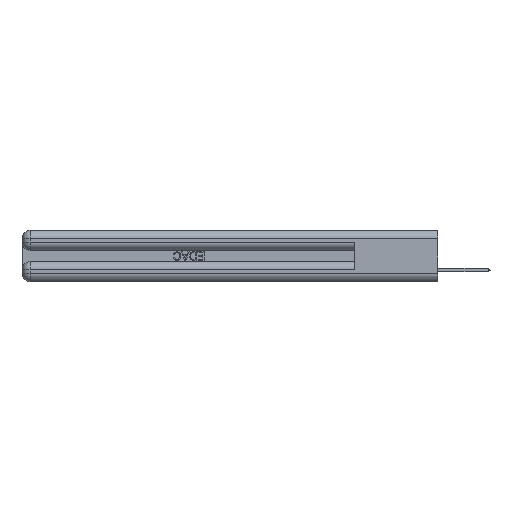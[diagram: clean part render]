
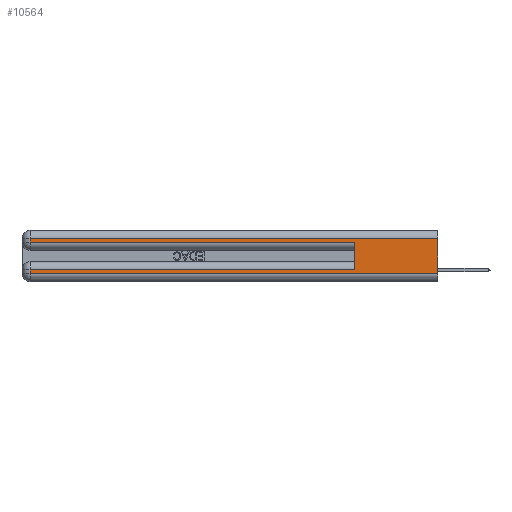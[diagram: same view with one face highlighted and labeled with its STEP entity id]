
A CAD part, left-side view. The second image highlights one B-rep face of the part: STEP entity #10564.
In plain terms, the highlighted planar face has unit normal (-1, 0, 0).
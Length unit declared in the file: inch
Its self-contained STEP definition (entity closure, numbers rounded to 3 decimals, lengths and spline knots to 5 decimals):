
#47 = VERTEX_POINT ( 'NONE', #4497 ) ;
#185 = EDGE_CURVE ( 'NONE', #15919, #32725, #11537, .T. ) ;
#721 = VERTEX_POINT ( 'NONE', #812 ) ;
#812 = CARTESIAN_POINT ( 'NONE',  ( 0., 0., 0.31 ) ) ;
#1434 = CARTESIAN_POINT ( 'NONE',  ( 0., 0., 0.31 ) ) ;
#1485 = VERTEX_POINT ( 'NONE', #38737 ) ;
#2323 = EDGE_CURVE ( 'NONE', #20501, #1485, #36766, .T. ) ;
#4497 = CARTESIAN_POINT ( 'NONE',  ( 0., 0., 0.06 ) ) ;
#5321 = VECTOR ( 'NONE', #28325, 39.37008 ) ;
#5468 = CARTESIAN_POINT ( 'NONE',  ( 0., 0., 0.06 ) ) ;
#7299 = LINE ( 'NONE', #14550, #41602 ) ;
#7753 = ORIENTED_EDGE ( 'NONE', *, *, #2323, .F. ) ;
#8168 = CARTESIAN_POINT ( 'NONE',  ( 0., 2.94, 0.085 ) ) ;
#10564 = ADVANCED_FACE ( 'NONE', ( #11035 ), #19225, .F. ) ;
#11035 = FACE_OUTER_BOUND ( 'NONE', #33458, .T. ) ;
#11233 = VECTOR ( 'NONE', #11423, 39.37008 ) ;
#11423 = DIRECTION ( 'NONE',  ( 0., 1., 0. ) ) ;
#11537 = LINE ( 'NONE', #41353, #5321 ) ;
#11681 = DIRECTION ( 'NONE',  ( 0., -1., 0. ) ) ;
#11895 = VERTEX_POINT ( 'NONE', #8168 ) ;
#13113 = CARTESIAN_POINT ( 'NONE',  ( 0., 2.94, 0.37 ) ) ;
#13334 = CARTESIAN_POINT ( 'NONE',  ( 0., 0., 0.285 ) ) ;
#14045 = LINE ( 'NONE', #33644, #32805 ) ;
#14369 = LINE ( 'NONE', #1434, #11233 ) ;
#14550 = CARTESIAN_POINT ( 'NONE',  ( 0., 0., 0.37 ) ) ;
#15776 = ORIENTED_EDGE ( 'NONE', *, *, #29492, .T. ) ;
#15919 = VERTEX_POINT ( 'NONE', #38553 ) ;
#16603 = CARTESIAN_POINT ( 'NONE',  ( 0., 0.6, 0.145 ) ) ;
#17990 = EDGE_CURVE ( 'NONE', #32725, #1485, #39197, .T. ) ;
#18737 = CARTESIAN_POINT ( 'NONE',  ( 0., 2.94, 0.285 ) ) ;
#19164 = VECTOR ( 'NONE', #11681, 39.37008 ) ;
#19225 = PLANE ( 'NONE',  #32962 ) ;
#19966 = ORIENTED_EDGE ( 'NONE', *, *, #39627, .F. ) ;
#20344 = ORIENTED_EDGE ( 'NONE', *, *, #20624, .T. ) ;
#20501 = VERTEX_POINT ( 'NONE', #36701 ) ;
#20624 = EDGE_CURVE ( 'NONE', #20501, #11895, #14045, .T. ) ;
#22515 = ORIENTED_EDGE ( 'NONE', *, *, #185, .T. ) ;
#24666 = VERTEX_POINT ( 'NONE', #39231 ) ;
#28325 = DIRECTION ( 'NONE',  ( 0., 0., -1. ) ) ;
#28877 = CARTESIAN_POINT ( 'NONE',  ( 0., 0., 0.37 ) ) ;
#29492 = EDGE_CURVE ( 'NONE', #721, #15919, #14369, .T. ) ;
#31294 = DIRECTION ( 'NONE',  ( 0., 0., -1. ) ) ;
#31740 = EDGE_CURVE ( 'NONE', #11895, #24666, #31829, .T. ) ;
#31829 = LINE ( 'NONE', #13113, #38002 ) ;
#32338 = ORIENTED_EDGE ( 'NONE', *, *, #31740, .T. ) ;
#32725 = VERTEX_POINT ( 'NONE', #18737 ) ;
#32805 = VECTOR ( 'NONE', #40495, 39.37008 ) ;
#32962 = AXIS2_PLACEMENT_3D ( 'NONE', #28877, #39152, #35523 ) ;
#33458 = EDGE_LOOP ( 'NONE', ( #19966, #15776, #22515, #36926, #7753, #20344, #32338, #38839 ) ) ;
#33644 = CARTESIAN_POINT ( 'NONE',  ( 0., 0., 0.085 ) ) ;
#33859 = EDGE_CURVE ( 'NONE', #24666, #47, #37883, .T. ) ;
#35238 = VECTOR ( 'NONE', #39918, 39.37008 ) ;
#35523 = DIRECTION ( 'NONE',  ( 0., 0., -1. ) ) ;
#36701 = CARTESIAN_POINT ( 'NONE',  ( 0., 0.6, 0.085 ) ) ;
#36766 = LINE ( 'NONE', #16603, #35238 ) ;
#36926 = ORIENTED_EDGE ( 'NONE', *, *, #17990, .T. ) ;
#37088 = VECTOR ( 'NONE', #40364, 39.37008 ) ;
#37883 = LINE ( 'NONE', #5468, #19164 ) ;
#38002 = VECTOR ( 'NONE', #40137, 39.37008 ) ;
#38553 = CARTESIAN_POINT ( 'NONE',  ( 0., 2.94, 0.31 ) ) ;
#38737 = CARTESIAN_POINT ( 'NONE',  ( 0., 0.6, 0.285 ) ) ;
#38839 = ORIENTED_EDGE ( 'NONE', *, *, #33859, .T. ) ;
#39152 = DIRECTION ( 'NONE',  ( 1., 0., 0. ) ) ;
#39197 = LINE ( 'NONE', #13334, #37088 ) ;
#39231 = CARTESIAN_POINT ( 'NONE',  ( 0., 2.94, 0.06 ) ) ;
#39627 = EDGE_CURVE ( 'NONE', #721, #47, #7299, .T. ) ;
#39918 = DIRECTION ( 'NONE',  ( 0., 0., 1. ) ) ;
#40137 = DIRECTION ( 'NONE',  ( 0., 0., -1. ) ) ;
#40364 = DIRECTION ( 'NONE',  ( 0., -1., 0. ) ) ;
#40495 = DIRECTION ( 'NONE',  ( 0., 1., 0. ) ) ;
#41353 = CARTESIAN_POINT ( 'NONE',  ( 0., 2.94, 0.37 ) ) ;
#41602 = VECTOR ( 'NONE', #31294, 39.37008 ) ;
